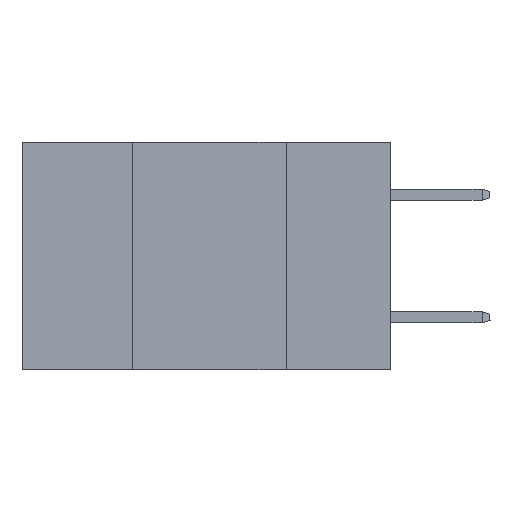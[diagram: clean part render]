
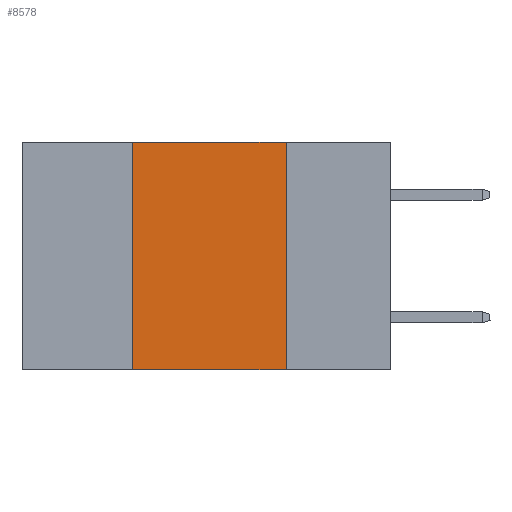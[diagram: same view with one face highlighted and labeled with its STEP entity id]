
A CAD part, left-side view. The second image highlights one B-rep face of the part: STEP entity #8578.
In plain terms, the highlighted planar face has unit normal (-1, 0, 0).
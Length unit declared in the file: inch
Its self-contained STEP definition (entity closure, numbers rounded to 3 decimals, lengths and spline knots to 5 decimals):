
#397 = CARTESIAN_POINT ( 'NONE',  ( 0., 0.6, 0. ) ) ;
#583 = VERTEX_POINT ( 'NONE', #11097 ) ;
#1555 = EDGE_CURVE ( 'NONE', #2020, #583, #7462, .T. ) ;
#1748 = FACE_OUTER_BOUND ( 'NONE', #10932, .T. ) ;
#2020 = VERTEX_POINT ( 'NONE', #6156 ) ;
#2424 = ORIENTED_EDGE ( 'NONE', *, *, #8959, .T. ) ;
#3026 = ORIENTED_EDGE ( 'NONE', *, *, #1555, .F. ) ;
#3377 = LINE ( 'NONE', #397, #11365 ) ;
#3905 = ORIENTED_EDGE ( 'NONE', *, *, #4293, .F. ) ;
#4060 = VERTEX_POINT ( 'NONE', #4561 ) ;
#4293 = EDGE_CURVE ( 'NONE', #4060, #11707, #8130, .T. ) ;
#4333 = DIRECTION ( 'NONE',  ( 0., -1., 0. ) ) ;
#4339 = AXIS2_PLACEMENT_3D ( 'NONE', #12321, #4469, #6658 ) ;
#4469 = DIRECTION ( 'NONE',  ( 1., 0., 0. ) ) ;
#4561 = CARTESIAN_POINT ( 'NONE',  ( 0., 0.17, 0. ) ) ;
#4573 = CARTESIAN_POINT ( 'NONE',  ( 0., 0.6, -0.37 ) ) ;
#4614 = VECTOR ( 'NONE', #10523, 39.37008 ) ;
#5893 = CARTESIAN_POINT ( 'NONE',  ( 0., 0.17, -0.37 ) ) ;
#6156 = CARTESIAN_POINT ( 'NONE',  ( 0., 0.42, -0.37 ) ) ;
#6583 = LINE ( 'NONE', #4573, #8687 ) ;
#6617 = ORIENTED_EDGE ( 'NONE', *, *, #8518, .F. ) ;
#6658 = DIRECTION ( 'NONE',  ( 0., 0., -1. ) ) ;
#7462 = LINE ( 'NONE', #10582, #4614 ) ;
#8130 = LINE ( 'NONE', #12012, #9203 ) ;
#8518 = EDGE_CURVE ( 'NONE', #583, #4060, #3377, .T. ) ;
#8578 = ADVANCED_FACE ( 'NONE', ( #1748 ), #12506, .F. ) ;
#8687 = VECTOR ( 'NONE', #12305, 39.37008 ) ;
#8959 = EDGE_CURVE ( 'NONE', #2020, #11707, #6583, .T. ) ;
#9203 = VECTOR ( 'NONE', #11880, 39.37008 ) ;
#10523 = DIRECTION ( 'NONE',  ( 0., 0., 1. ) ) ;
#10582 = CARTESIAN_POINT ( 'NONE',  ( 0., 0.42, 0. ) ) ;
#10932 = EDGE_LOOP ( 'NONE', ( #3905, #6617, #3026, #2424 ) ) ;
#11097 = CARTESIAN_POINT ( 'NONE',  ( 0., 0.42, 0. ) ) ;
#11365 = VECTOR ( 'NONE', #4333, 39.37008 ) ;
#11707 = VERTEX_POINT ( 'NONE', #5893 ) ;
#11880 = DIRECTION ( 'NONE',  ( 0., 0., -1. ) ) ;
#12012 = CARTESIAN_POINT ( 'NONE',  ( 0., 0.17, 0. ) ) ;
#12305 = DIRECTION ( 'NONE',  ( 0., -1., 0. ) ) ;
#12321 = CARTESIAN_POINT ( 'NONE',  ( 0., 0.6, 0. ) ) ;
#12506 = PLANE ( 'NONE',  #4339 ) ;
